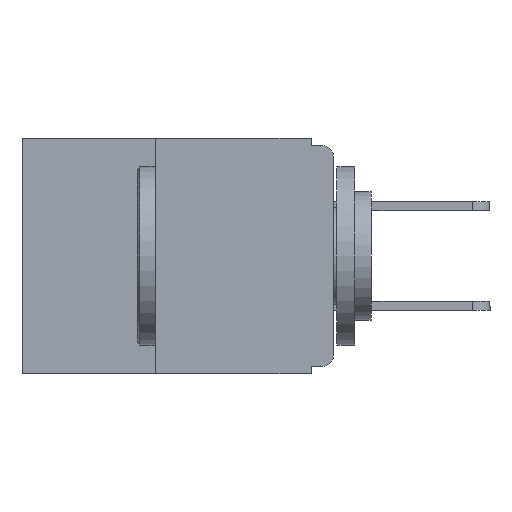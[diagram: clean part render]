
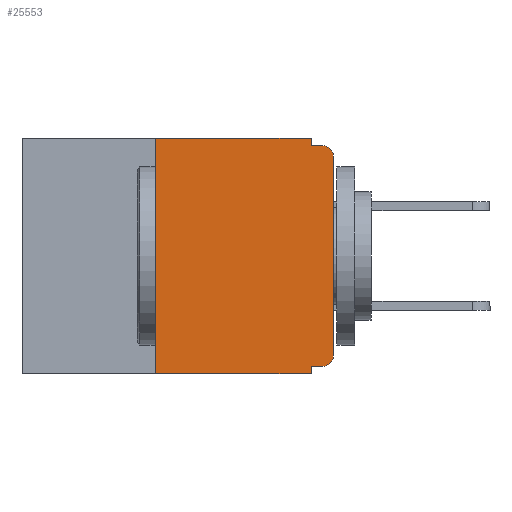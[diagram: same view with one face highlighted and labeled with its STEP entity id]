
A CAD part, left-side view. The second image highlights one B-rep face of the part: STEP entity #25553.
In plain terms, the highlighted planar face has unit normal (-1, 0, 0).
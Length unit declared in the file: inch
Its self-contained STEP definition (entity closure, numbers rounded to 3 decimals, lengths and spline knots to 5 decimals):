
#369 = CARTESIAN_POINT ( 'NONE',  ( 0., 0.437, 0. ) ) ;
#709 = EDGE_CURVE ( 'NONE', #24441, #8058, #26246, .T. ) ;
#735 = CARTESIAN_POINT ( 'NONE',  ( 0., 0.437, 0. ) ) ;
#789 = ORIENTED_EDGE ( 'NONE', *, *, #7281, .T. ) ;
#860 = AXIS2_PLACEMENT_3D ( 'NONE', #16668, #4070, #18820 ) ;
#891 = DIRECTION ( 'NONE',  ( -1., 0., 0. ) ) ;
#2002 = DIRECTION ( 'NONE',  ( 0., -1., 0. ) ) ;
#2119 = VERTEX_POINT ( 'NONE', #5493 ) ;
#2572 = DIRECTION ( 'NONE',  ( 0., 0., -1. ) ) ;
#3344 = CARTESIAN_POINT ( 'NONE',  ( 0., 0.437, -0.33 ) ) ;
#4062 = VERTEX_POINT ( 'NONE', #7123 ) ;
#4070 = DIRECTION ( 'NONE',  ( -1., 0., 0. ) ) ;
#4704 = VERTEX_POINT ( 'NONE', #4917 ) ;
#4917 = CARTESIAN_POINT ( 'NONE',  ( 0., 0.25, -0.33 ) ) ;
#5073 = ORIENTED_EDGE ( 'NONE', *, *, #26657, .T. ) ;
#5176 = VECTOR ( 'NONE', #9626, 39.37008 ) ;
#5493 = CARTESIAN_POINT ( 'NONE',  ( 0., 0.25, 0. ) ) ;
#5848 = ORIENTED_EDGE ( 'NONE', *, *, #7958, .T. ) ;
#6144 = CARTESIAN_POINT ( 'NONE',  ( 0., 0., -0.01 ) ) ;
#6157 = CARTESIAN_POINT ( 'NONE',  ( 0., 0.031, -0.33 ) ) ;
#7123 = CARTESIAN_POINT ( 'NONE',  ( 0., 0.015, -0.32 ) ) ;
#7281 = EDGE_CURVE ( 'NONE', #23876, #26360, #24791, .T. ) ;
#7527 = CARTESIAN_POINT ( 'NONE',  ( 0., 0.031, 0. ) ) ;
#7735 = ORIENTED_EDGE ( 'NONE', *, *, #17011, .F. ) ;
#7958 = EDGE_CURVE ( 'NONE', #4704, #17524, #13421, .T. ) ;
#8058 = VERTEX_POINT ( 'NONE', #14181 ) ;
#8452 = VECTOR ( 'NONE', #18103, 39.37008 ) ;
#9626 = DIRECTION ( 'NONE',  ( 0., 0., -1. ) ) ;
#9677 = EDGE_CURVE ( 'NONE', #4704, #2119, #10973, .T. ) ;
#9888 = VECTOR ( 'NONE', #15930, 39.37008 ) ;
#10761 = LINE ( 'NONE', #7527, #5176 ) ;
#10973 = LINE ( 'NONE', #22677, #21520 ) ;
#10976 = EDGE_CURVE ( 'NONE', #14303, #17524, #21084, .T. ) ;
#11139 = CARTESIAN_POINT ( 'NONE',  ( 0., 0., 0. ) ) ;
#12337 = DIRECTION ( 'NONE',  ( 0., 0., 1. ) ) ;
#12925 = VERTEX_POINT ( 'NONE', #22406 ) ;
#13192 = CARTESIAN_POINT ( 'NONE',  ( 0., 0.031, -0.33 ) ) ;
#13421 = LINE ( 'NONE', #3344, #8452 ) ;
#13541 = CARTESIAN_POINT ( 'NONE',  ( 0., 0., -0.305 ) ) ;
#13556 = CIRCLE ( 'NONE', #860, 0.015 ) ;
#13584 = FACE_OUTER_BOUND ( 'NONE', #23860, .T. ) ;
#13661 = CARTESIAN_POINT ( 'NONE',  ( 0., 0.015, -0.025 ) ) ;
#13863 = CARTESIAN_POINT ( 'NONE',  ( 0., 0., -0.32 ) ) ;
#14094 = AXIS2_PLACEMENT_3D ( 'NONE', #13661, #891, #15723 ) ;
#14181 = CARTESIAN_POINT ( 'NONE',  ( 0., 0.015, -0.01 ) ) ;
#14303 = VERTEX_POINT ( 'NONE', #24593 ) ;
#14766 = ORIENTED_EDGE ( 'NONE', *, *, #16343, .F. ) ;
#14881 = VECTOR ( 'NONE', #17713, 39.37008 ) ;
#15007 = ORIENTED_EDGE ( 'NONE', *, *, #26001, .T. ) ;
#15071 = VECTOR ( 'NONE', #25636, 39.37008 ) ;
#15237 = DIRECTION ( 'NONE',  ( 1., 0., 0. ) ) ;
#15723 = DIRECTION ( 'NONE',  ( 0., 0., -1. ) ) ;
#15930 = DIRECTION ( 'NONE',  ( 0., 1., 0. ) ) ;
#16343 = EDGE_CURVE ( 'NONE', #2119, #12925, #20490, .T. ) ;
#16668 = CARTESIAN_POINT ( 'NONE',  ( 0., 0.015, -0.305 ) ) ;
#17011 = EDGE_CURVE ( 'NONE', #4062, #14303, #20452, .T. ) ;
#17524 = VERTEX_POINT ( 'NONE', #13192 ) ;
#17713 = DIRECTION ( 'NONE',  ( 0., -1., 0. ) ) ;
#17854 = ORIENTED_EDGE ( 'NONE', *, *, #9677, .F. ) ;
#18103 = DIRECTION ( 'NONE',  ( 0., -1., 0. ) ) ;
#18281 = ORIENTED_EDGE ( 'NONE', *, *, #709, .F. ) ;
#18820 = DIRECTION ( 'NONE',  ( 0., 0., -1. ) ) ;
#19237 = ORIENTED_EDGE ( 'NONE', *, *, #19769, .F. ) ;
#19769 = EDGE_CURVE ( 'NONE', #12925, #24441, #10761, .T. ) ;
#20409 = AXIS2_PLACEMENT_3D ( 'NONE', #369, #15237, #2572 ) ;
#20452 = LINE ( 'NONE', #13863, #9888 ) ;
#20490 = LINE ( 'NONE', #735, #14881 ) ;
#20903 = DIRECTION ( 'NONE',  ( 0., 0., -1. ) ) ;
#21084 = LINE ( 'NONE', #6157, #26412 ) ;
#21520 = VECTOR ( 'NONE', #12337, 39.37008 ) ;
#21564 = VECTOR ( 'NONE', #2002, 39.37008 ) ;
#22406 = CARTESIAN_POINT ( 'NONE',  ( 0., 0.031, 0. ) ) ;
#22677 = CARTESIAN_POINT ( 'NONE',  ( 0., 0.25, -0.33 ) ) ;
#23465 = PLANE ( 'NONE',  #20409 ) ;
#23860 = EDGE_LOOP ( 'NONE', ( #789, #5073, #18281, #19237, #14766, #17854, #5848, #26085, #7735, #15007 ) ) ;
#23876 = VERTEX_POINT ( 'NONE', #13541 ) ;
#24039 = CARTESIAN_POINT ( 'NONE',  ( 0., 0., -0.025 ) ) ;
#24441 = VERTEX_POINT ( 'NONE', #25832 ) ;
#24593 = CARTESIAN_POINT ( 'NONE',  ( 0., 0.031, -0.32 ) ) ;
#24791 = LINE ( 'NONE', #11139, #15071 ) ;
#24845 = CIRCLE ( 'NONE', #14094, 0.015 ) ;
#25553 = ADVANCED_FACE ( 'NONE', ( #13584 ), #23465, .F. ) ;
#25636 = DIRECTION ( 'NONE',  ( 0., 0., 1. ) ) ;
#25832 = CARTESIAN_POINT ( 'NONE',  ( 0., 0.031, -0.01 ) ) ;
#26001 = EDGE_CURVE ( 'NONE', #4062, #23876, #13556, .T. ) ;
#26085 = ORIENTED_EDGE ( 'NONE', *, *, #10976, .F. ) ;
#26246 = LINE ( 'NONE', #6144, #21564 ) ;
#26360 = VERTEX_POINT ( 'NONE', #24039 ) ;
#26412 = VECTOR ( 'NONE', #20903, 39.37008 ) ;
#26657 = EDGE_CURVE ( 'NONE', #26360, #8058, #24845, .T. ) ;
